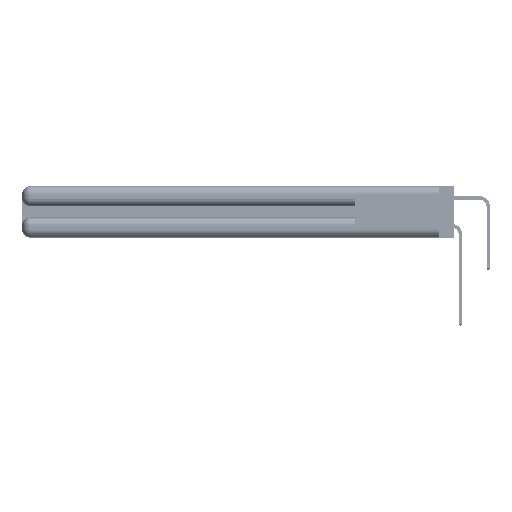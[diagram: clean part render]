
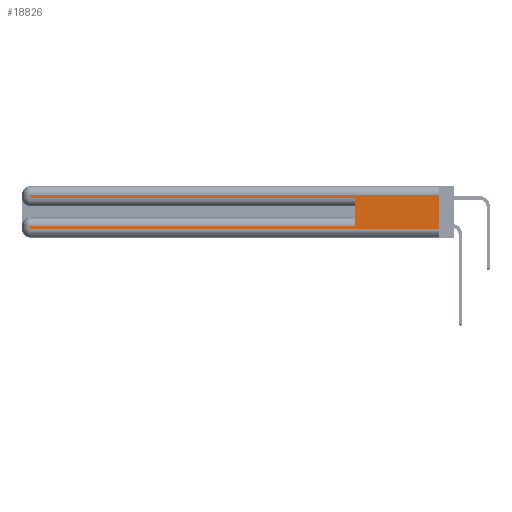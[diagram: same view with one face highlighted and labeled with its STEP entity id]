
A CAD part, left-side view. The second image highlights one B-rep face of the part: STEP entity #18826.
In plain terms, the highlighted planar face has unit normal (-1, 0, 0).
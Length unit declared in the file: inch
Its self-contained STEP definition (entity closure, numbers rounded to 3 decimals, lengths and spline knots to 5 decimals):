
#633 = VERTEX_POINT ( 'NONE', #50951 ) ;
#2590 = DIRECTION ( 'NONE',  ( 0., 0., -1. ) ) ;
#3447 = VERTEX_POINT ( 'NONE', #12176 ) ;
#4867 = EDGE_CURVE ( 'NONE', #27069, #15235, #31162, .T. ) ;
#6902 = CARTESIAN_POINT ( 'NONE',  ( 0., 0., 0.085 ) ) ;
#7158 = CARTESIAN_POINT ( 'NONE',  ( 0., 0., 0.06 ) ) ;
#7821 = LINE ( 'NONE', #37048, #26741 ) ;
#7978 = VERTEX_POINT ( 'NONE', #7158 ) ;
#8005 = FACE_OUTER_BOUND ( 'NONE', #22375, .T. ) ;
#8112 = EDGE_CURVE ( 'NONE', #12202, #633, #31703, .T. ) ;
#8280 = CARTESIAN_POINT ( 'NONE',  ( 0., 0., 0.31 ) ) ;
#8433 = EDGE_CURVE ( 'NONE', #39416, #48479, #48292, .T. ) ;
#9884 = CARTESIAN_POINT ( 'NONE',  ( 0., 2.94, 0.31 ) ) ;
#10579 = VECTOR ( 'NONE', #37231, 39.37008 ) ;
#11175 = CARTESIAN_POINT ( 'NONE',  ( 0., 2.94, 0.085 ) ) ;
#12054 = DIRECTION ( 'NONE',  ( 0., 0., -1. ) ) ;
#12176 = CARTESIAN_POINT ( 'NONE',  ( 0., 0., 0.31 ) ) ;
#12202 = VERTEX_POINT ( 'NONE', #13881 ) ;
#12579 = CARTESIAN_POINT ( 'NONE',  ( 0., 2.94, 0.06 ) ) ;
#12642 = DIRECTION ( 'NONE',  ( 0., 1., 0. ) ) ;
#13101 = LINE ( 'NONE', #8280, #34599 ) ;
#13881 = CARTESIAN_POINT ( 'NONE',  ( 0., 0.6, 0.085 ) ) ;
#15235 = VERTEX_POINT ( 'NONE', #45699 ) ;
#15332 = ORIENTED_EDGE ( 'NONE', *, *, #49780, .T. ) ;
#16705 = ORIENTED_EDGE ( 'NONE', *, *, #4867, .T. ) ;
#16761 = ORIENTED_EDGE ( 'NONE', *, *, #8433, .T. ) ;
#17830 = CARTESIAN_POINT ( 'NONE',  ( 0., 0., 0.37 ) ) ;
#18414 = LINE ( 'NONE', #6902, #28490 ) ;
#18805 = ORIENTED_EDGE ( 'NONE', *, *, #8112, .F. ) ;
#18826 = ADVANCED_FACE ( 'NONE', ( #8005 ), #43389, .F. ) ;
#19196 = EDGE_CURVE ( 'NONE', #3447, #7978, #7821, .T. ) ;
#20835 = ORIENTED_EDGE ( 'NONE', *, *, #47277, .T. ) ;
#21022 = CARTESIAN_POINT ( 'NONE',  ( 0., 0.6, 0.145 ) ) ;
#21055 = LINE ( 'NONE', #47508, #42363 ) ;
#22211 = DIRECTION ( 'NONE',  ( 1., 0., 0. ) ) ;
#22375 = EDGE_LOOP ( 'NONE', ( #40103, #15332, #16705, #20835, #18805, #55474, #16761, #31477 ) ) ;
#24830 = LINE ( 'NONE', #50072, #10579 ) ;
#25118 = CARTESIAN_POINT ( 'NONE',  ( 0., 2.94, 0.37 ) ) ;
#26741 = VECTOR ( 'NONE', #2590, 39.37008 ) ;
#27069 = VERTEX_POINT ( 'NONE', #9884 ) ;
#27160 = DIRECTION ( 'NONE',  ( 0., 0., -1. ) ) ;
#28490 = VECTOR ( 'NONE', #41241, 39.37008 ) ;
#31162 = LINE ( 'NONE', #25118, #41109 ) ;
#31477 = ORIENTED_EDGE ( 'NONE', *, *, #45059, .T. ) ;
#31703 = LINE ( 'NONE', #21022, #41644 ) ;
#33343 = EDGE_CURVE ( 'NONE', #12202, #39416, #18414, .T. ) ;
#34599 = VECTOR ( 'NONE', #12642, 39.37008 ) ;
#37048 = CARTESIAN_POINT ( 'NONE',  ( 0., 0., 0.37 ) ) ;
#37231 = DIRECTION ( 'NONE',  ( 0., -1., 0. ) ) ;
#39416 = VERTEX_POINT ( 'NONE', #11175 ) ;
#40103 = ORIENTED_EDGE ( 'NONE', *, *, #19196, .F. ) ;
#41109 = VECTOR ( 'NONE', #12054, 39.37008 ) ;
#41241 = DIRECTION ( 'NONE',  ( 0., 1., 0. ) ) ;
#41644 = VECTOR ( 'NONE', #55065, 39.37008 ) ;
#42363 = VECTOR ( 'NONE', #51783, 39.37008 ) ;
#43389 = PLANE ( 'NONE',  #51201 ) ;
#45059 = EDGE_CURVE ( 'NONE', #48479, #7978, #21055, .T. ) ;
#45699 = CARTESIAN_POINT ( 'NONE',  ( 0., 2.94, 0.285 ) ) ;
#46956 = VECTOR ( 'NONE', #27160, 39.37008 ) ;
#47277 = EDGE_CURVE ( 'NONE', #15235, #633, #24830, .T. ) ;
#47508 = CARTESIAN_POINT ( 'NONE',  ( 0., 0., 0.06 ) ) ;
#48292 = LINE ( 'NONE', #52811, #46956 ) ;
#48479 = VERTEX_POINT ( 'NONE', #12579 ) ;
#49780 = EDGE_CURVE ( 'NONE', #3447, #27069, #13101, .T. ) ;
#50072 = CARTESIAN_POINT ( 'NONE',  ( 0., 0., 0.285 ) ) ;
#50951 = CARTESIAN_POINT ( 'NONE',  ( 0., 0.6, 0.285 ) ) ;
#51201 = AXIS2_PLACEMENT_3D ( 'NONE', #17830, #22211, #51957 ) ;
#51783 = DIRECTION ( 'NONE',  ( 0., -1., 0. ) ) ;
#51957 = DIRECTION ( 'NONE',  ( 0., 0., -1. ) ) ;
#52811 = CARTESIAN_POINT ( 'NONE',  ( 0., 2.94, 0.37 ) ) ;
#55065 = DIRECTION ( 'NONE',  ( 0., 0., 1. ) ) ;
#55474 = ORIENTED_EDGE ( 'NONE', *, *, #33343, .T. ) ;
